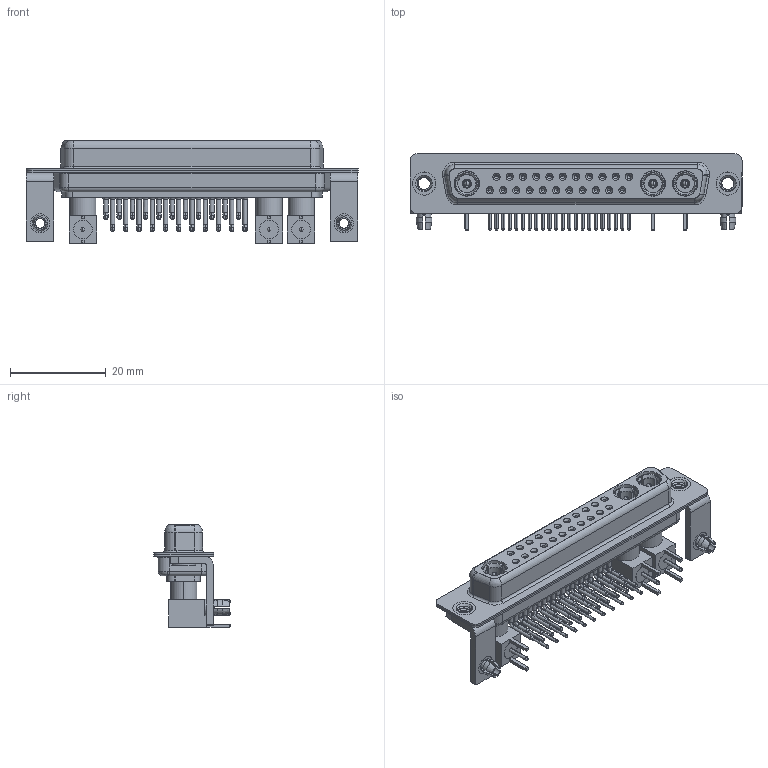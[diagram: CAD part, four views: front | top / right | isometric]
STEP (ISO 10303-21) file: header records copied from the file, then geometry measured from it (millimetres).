
FILE_DESCRIPTION (( 'STEP AP203' ), '1' );
FILE_NAME ('630-25W3240-7TB.STEP', '2022-06-07T04:24:14', ( '' ), ( '' ), 'SwSTEP 2.0', 'SolidWorks 2020', '' );
FILE_SCHEMA (( 'CONFIG_CONTROL_DESIGN' ));
Length unit declared in the file: millimetre
Products named in the file (18): 630Combo Contact Row 2; 630Combo Contact Row 1; 630-25W3240-7TB; Insulator RA Pin; Co-Ax Plug Assy_RA; Co-Ax Plug_RA PC Tail; Locking Collar; 630Combo Threaded Rivet_B; 630Combo Shell Front_37 Contacts; Insulator Pin_Straight PC Tail; RA Back Shell; 630Combo Stabilizer Bracket; 630Combo Housing_25W3; 630Combo Shell Rear_37 Contacts; 630Combo Board Lock; Pin_RA
Assembly tree (52 placements, depth 3):
  630-25W3240-7TB
    630Combo Housing_25W3
    630Combo Shell Front_37 Contacts
    630Combo Shell Rear_37 Contacts
    630Combo Threaded Rivet_B  x2
    630Combo Stabilizer Bracket  x2
    630Combo Board Lock  x2
    Co-Ax Plug Assy_RA
      Co-Ax Plug_RA PC Tail
      Insulator Pin_Straight PC Tail
      Pin_RA
      Locking Collar
      RA Back Shell
      Insulator RA Pin
    Co-Ax Plug Assy_RA
      Co-Ax Plug_RA PC Tail
      Insulator Pin_Straight PC Tail
      Pin_RA
      Locking Collar
      RA Back Shell
      Insulator RA Pin
    Co-Ax Plug Assy_RA
      Co-Ax Plug_RA PC Tail
      Insulator Pin_Straight PC Tail
      Pin_RA
      Locking Collar
      RA Back Shell
      Insulator RA Pin
    630Combo Contact Row 1  x11
    630Combo Contact Row 2  x11
Bounding box: 69.4 x 16 x 21.41 mm (x, y, z)
Volume: 6471.1 mm3; surface area: 15378.5 mm2
Topology: 49 solids, 49 shells, 2079 faces, 5202 edges, 3276 vertices
Faces by surface type: cylinder 888, plane 666, cone 341, bspline 97, torus 75, sphere 12
Entity records: 29778 total; most frequent: CARTESIAN_POINT 6266, DIRECTION 4745, ORIENTED_EDGE 4022, EDGE_CURVE 2011, AXIS2_PLACEMENT_3D 1952, VERTEX_POINT 1283, CIRCLE 1051, EDGE_LOOP 1032
